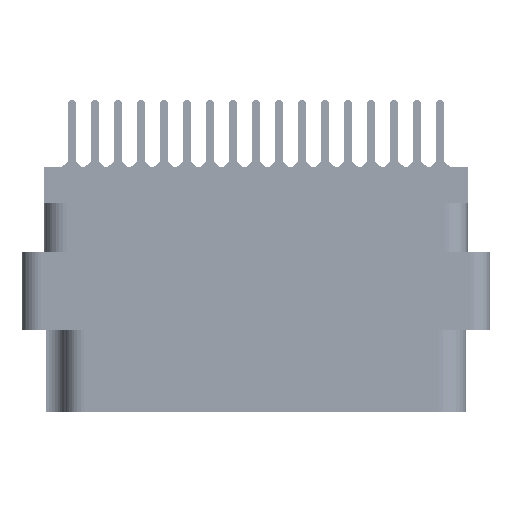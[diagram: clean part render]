
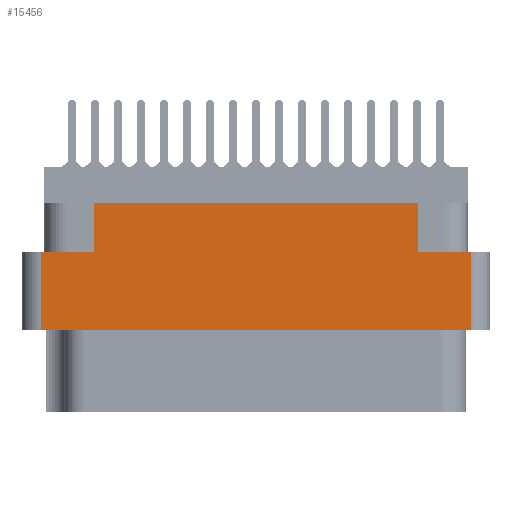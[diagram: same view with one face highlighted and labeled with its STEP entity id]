
A CAD part, left-side view. The second image highlights one B-rep face of the part: STEP entity #15456.
In plain terms, the highlighted planar face has unit normal (-1, 0, 0).
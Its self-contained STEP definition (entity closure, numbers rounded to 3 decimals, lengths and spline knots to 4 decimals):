
#1022 = CARTESIAN_POINT ( 'NONE',  ( -1.375, -0.7005, -0.529 ) ) ;
#4838 = VECTOR ( 'NONE', #59882, 39.3701 ) ;
#5578 = DIRECTION ( 'NONE',  ( 0., 0., 1. ) ) ;
#6102 = CARTESIAN_POINT ( 'NONE',  ( -1.375, 0.5285, -0.117 ) ) ;
#6193 = PLANE ( 'NONE',  #55388 ) ;
#6517 = DIRECTION ( 'NONE',  ( -1., 0., 0. ) ) ;
#10817 = CARTESIAN_POINT ( 'NONE',  ( -1.375, 0.7625, -0.117 ) ) ;
#11694 = CARTESIAN_POINT ( 'NONE',  ( -1.375, 0.7005, -0.529 ) ) ;
#12595 = DIRECTION ( 'NONE',  ( 0., 1., 0. ) ) ;
#12628 = CARTESIAN_POINT ( 'NONE',  ( -1.375, 0.7005, -0.277 ) ) ;
#13493 = CARTESIAN_POINT ( 'NONE',  ( -1.375, -0.7625, -0.798 ) ) ;
#14557 = EDGE_CURVE ( 'NONE', #48404, #66997, #30680, .T. ) ;
#15456 = ADVANCED_FACE ( 'NONE', ( #58882 ), #6193, .T. ) ;
#15538 = CARTESIAN_POINT ( 'NONE',  ( -1.375, 0.7005, -0.798 ) ) ;
#17343 = CARTESIAN_POINT ( 'NONE',  ( -1.375, 0.5285, -0.277 ) ) ;
#17935 = VERTEX_POINT ( 'NONE', #63279 ) ;
#19203 = VECTOR ( 'NONE', #71053, 39.3701 ) ;
#20528 = CARTESIAN_POINT ( 'NONE',  ( -1.375, 0., -0.529 ) ) ;
#21385 = VECTOR ( 'NONE', #24983, 39.3701 ) ;
#24983 = DIRECTION ( 'NONE',  ( 0., 0., 1. ) ) ;
#25302 = CARTESIAN_POINT ( 'NONE',  ( -1.375, -0.5285, -0.277 ) ) ;
#25425 = LINE ( 'NONE', #72272, #4838 ) ;
#27466 = EDGE_CURVE ( 'NONE', #66997, #32162, #25425, .T. ) ;
#30680 = LINE ( 'NONE', #48641, #52187 ) ;
#31154 = VECTOR ( 'NONE', #54328, 39.3701 ) ;
#31772 = LINE ( 'NONE', #48813, #19203 ) ;
#32159 = EDGE_LOOP ( 'NONE', ( #89407, #80333, #93507, #61722, #65123, #55926, #55876, #37066 ) ) ;
#32162 = VERTEX_POINT ( 'NONE', #6102 ) ;
#33741 = EDGE_CURVE ( 'NONE', #78653, #52136, #65456, .T. ) ;
#34511 = LINE ( 'NONE', #10817, #31154 ) ;
#37066 = ORIENTED_EDGE ( 'NONE', *, *, #27466, .F. ) ;
#39313 = VECTOR ( 'NONE', #12595, 39.3701 ) ;
#39473 = DIRECTION ( 'NONE',  ( 0., 0., 1. ) ) ;
#39940 = EDGE_CURVE ( 'NONE', #17935, #86629, #31772, .T. ) ;
#40815 = LINE ( 'NONE', #68355, #61259 ) ;
#43616 = VERTEX_POINT ( 'NONE', #75349 ) ;
#43714 = EDGE_CURVE ( 'NONE', #32162, #43616, #34511, .T. ) ;
#48404 = VERTEX_POINT ( 'NONE', #12628 ) ;
#48641 = CARTESIAN_POINT ( 'NONE',  ( -1.375, 0., -0.277 ) ) ;
#48813 = CARTESIAN_POINT ( 'NONE',  ( -1.375, 0., -0.277 ) ) ;
#50371 = EDGE_CURVE ( 'NONE', #48404, #52136, #61595, .T. ) ;
#52136 = VERTEX_POINT ( 'NONE', #11694 ) ;
#52187 = VECTOR ( 'NONE', #93083, 39.3701 ) ;
#54256 = DIRECTION ( 'NONE',  ( 0., 0., -1. ) ) ;
#54328 = DIRECTION ( 'NONE',  ( 0., -1., 0. ) ) ;
#55388 = AXIS2_PLACEMENT_3D ( 'NONE', #13493, #6517, #5578 ) ;
#55876 = ORIENTED_EDGE ( 'NONE', *, *, #43714, .F. ) ;
#55926 = ORIENTED_EDGE ( 'NONE', *, *, #71416, .T. ) ;
#56991 = CARTESIAN_POINT ( 'NONE',  ( -1.375, -0.7005, -0.277 ) ) ;
#58882 = FACE_OUTER_BOUND ( 'NONE', #32159, .T. ) ;
#59882 = DIRECTION ( 'NONE',  ( 0., 0., 1. ) ) ;
#61259 = VECTOR ( 'NONE', #39473, 39.3701 ) ;
#61480 = EDGE_CURVE ( 'NONE', #78653, #86629, #40815, .T. ) ;
#61595 = LINE ( 'NONE', #15538, #75247 ) ;
#61722 = ORIENTED_EDGE ( 'NONE', *, *, #61480, .T. ) ;
#63279 = CARTESIAN_POINT ( 'NONE',  ( -1.375, -0.5285, -0.277 ) ) ;
#65123 = ORIENTED_EDGE ( 'NONE', *, *, #39940, .F. ) ;
#65456 = LINE ( 'NONE', #20528, #39313 ) ;
#66997 = VERTEX_POINT ( 'NONE', #17343 ) ;
#68355 = CARTESIAN_POINT ( 'NONE',  ( -1.375, -0.7005, -0.798 ) ) ;
#71053 = DIRECTION ( 'NONE',  ( 0., -1., 0. ) ) ;
#71416 = EDGE_CURVE ( 'NONE', #17935, #43616, #81600, .T. ) ;
#72272 = CARTESIAN_POINT ( 'NONE',  ( -1.375, 0.5285, -0.277 ) ) ;
#75247 = VECTOR ( 'NONE', #54256, 39.3701 ) ;
#75349 = CARTESIAN_POINT ( 'NONE',  ( -1.375, -0.5285, -0.117 ) ) ;
#78653 = VERTEX_POINT ( 'NONE', #1022 ) ;
#80333 = ORIENTED_EDGE ( 'NONE', *, *, #50371, .T. ) ;
#81600 = LINE ( 'NONE', #25302, #21385 ) ;
#86629 = VERTEX_POINT ( 'NONE', #56991 ) ;
#89407 = ORIENTED_EDGE ( 'NONE', *, *, #14557, .F. ) ;
#93083 = DIRECTION ( 'NONE',  ( 0., -1., 0. ) ) ;
#93507 = ORIENTED_EDGE ( 'NONE', *, *, #33741, .F. ) ;
